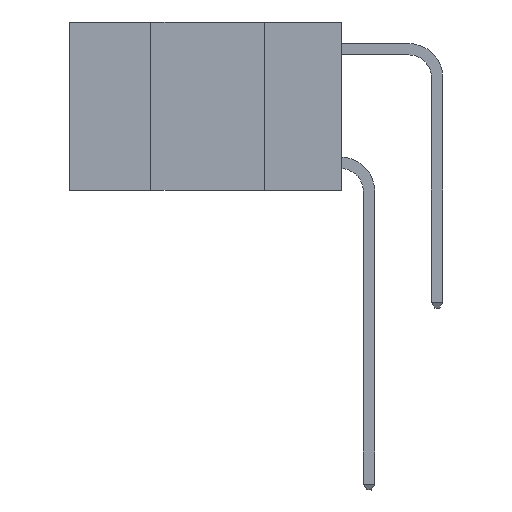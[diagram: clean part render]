
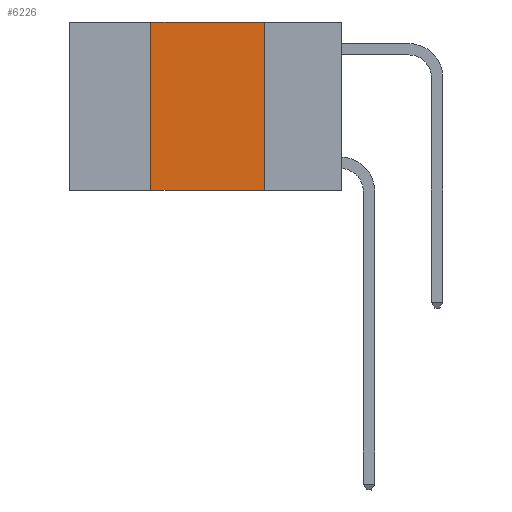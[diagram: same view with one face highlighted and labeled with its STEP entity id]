
A CAD part, left-side view. The second image highlights one B-rep face of the part: STEP entity #6226.
In plain terms, the highlighted planar face has unit normal (-1, 0, 0).
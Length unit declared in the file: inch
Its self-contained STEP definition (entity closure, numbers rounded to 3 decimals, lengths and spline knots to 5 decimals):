
#592 = VECTOR ( 'NONE', #6360, 39.37008 ) ;
#902 = ORIENTED_EDGE ( 'NONE', *, *, #3149, .F. ) ;
#922 = ORIENTED_EDGE ( 'NONE', *, *, #5644, .F. ) ;
#1273 = EDGE_CURVE ( 'NONE', #5885, #10645, #5867, .T. ) ;
#1981 = ORIENTED_EDGE ( 'NONE', *, *, #5332, .T. ) ;
#2155 = CARTESIAN_POINT ( 'NONE',  ( 0., 0.42, -0.37 ) ) ;
#2520 = DIRECTION ( 'NONE',  ( 0., 0., 1. ) ) ;
#2739 = FACE_OUTER_BOUND ( 'NONE', #10152, .T. ) ;
#2876 = VECTOR ( 'NONE', #7400, 39.37008 ) ;
#3149 = EDGE_CURVE ( 'NONE', #6311, #5885, #6955, .T. ) ;
#3400 = LINE ( 'NONE', #6670, #5816 ) ;
#3496 = CARTESIAN_POINT ( 'NONE',  ( 0., 0.42, 0. ) ) ;
#3505 = CARTESIAN_POINT ( 'NONE',  ( 0., 0.6, 0. ) ) ;
#3564 = PLANE ( 'NONE',  #7149 ) ;
#3888 = VERTEX_POINT ( 'NONE', #8200 ) ;
#3901 = DIRECTION ( 'NONE',  ( 0., -1., 0. ) ) ;
#4459 = DIRECTION ( 'NONE',  ( 1., 0., 0. ) ) ;
#5332 = EDGE_CURVE ( 'NONE', #6311, #3888, #3400, .T. ) ;
#5644 = EDGE_CURVE ( 'NONE', #10645, #3888, #9767, .T. ) ;
#5774 = ORIENTED_EDGE ( 'NONE', *, *, #1273, .F. ) ;
#5816 = VECTOR ( 'NONE', #3901, 39.37008 ) ;
#5867 = LINE ( 'NONE', #3505, #592 ) ;
#5885 = VERTEX_POINT ( 'NONE', #3496 ) ;
#6226 = ADVANCED_FACE ( 'NONE', ( #2739 ), #3564, .F. ) ;
#6311 = VERTEX_POINT ( 'NONE', #2155 ) ;
#6360 = DIRECTION ( 'NONE',  ( 0., -1., 0. ) ) ;
#6670 = CARTESIAN_POINT ( 'NONE',  ( 0., 0.6, -0.37 ) ) ;
#6955 = LINE ( 'NONE', #7221, #11122 ) ;
#7149 = AXIS2_PLACEMENT_3D ( 'NONE', #8802, #4459, #10531 ) ;
#7221 = CARTESIAN_POINT ( 'NONE',  ( 0., 0.42, 0. ) ) ;
#7400 = DIRECTION ( 'NONE',  ( 0., 0., -1. ) ) ;
#8200 = CARTESIAN_POINT ( 'NONE',  ( 0., 0.17, -0.37 ) ) ;
#8802 = CARTESIAN_POINT ( 'NONE',  ( 0., 0.6, 0. ) ) ;
#8918 = CARTESIAN_POINT ( 'NONE',  ( 0., 0.17, 0. ) ) ;
#9039 = CARTESIAN_POINT ( 'NONE',  ( 0., 0.17, 0. ) ) ;
#9767 = LINE ( 'NONE', #9039, #2876 ) ;
#10152 = EDGE_LOOP ( 'NONE', ( #922, #5774, #902, #1981 ) ) ;
#10531 = DIRECTION ( 'NONE',  ( 0., 0., -1. ) ) ;
#10645 = VERTEX_POINT ( 'NONE', #8918 ) ;
#11122 = VECTOR ( 'NONE', #2520, 39.37008 ) ;
